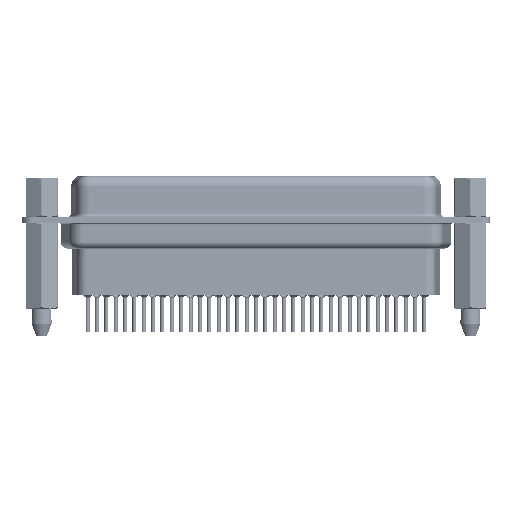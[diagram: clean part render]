
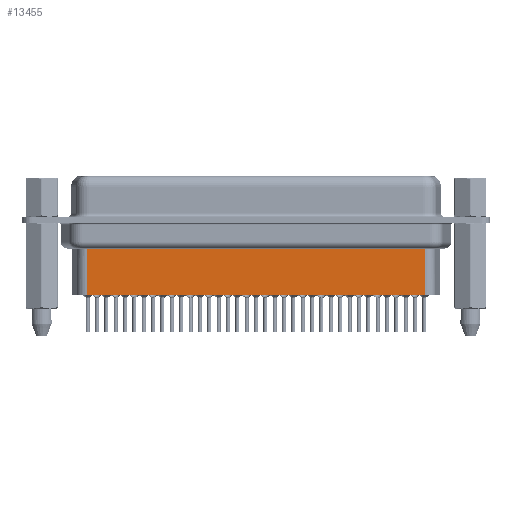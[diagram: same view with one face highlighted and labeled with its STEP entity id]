
A CAD part, front view. The second image highlights one B-rep face of the part: STEP entity #13455.
In plain terms, the highlighted planar face has unit normal (0, -1, 0).
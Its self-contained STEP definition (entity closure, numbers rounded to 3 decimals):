
#144 = CARTESIAN_POINT ( 'NONE',  ( 56.794, -3.5, -4.097 ) ) ;
#350 = VERTEX_POINT ( 'NONE', #13398 ) ;
#1258 = VECTOR ( 'NONE', #24046, 1000. ) ;
#1282 = DIRECTION ( 'NONE',  ( 1., 0., 0. ) ) ;
#3902 = DIRECTION ( 'NONE',  ( 0., 0., -1. ) ) ;
#7514 = EDGE_CURVE ( 'NONE', #37423, #31630, #21726, .T. ) ;
#7929 = AXIS2_PLACEMENT_3D ( 'NONE', #31589, #13810, #1282 ) ;
#12096 = LINE ( 'NONE', #15792, #1258 ) ;
#13398 = CARTESIAN_POINT ( 'NONE',  ( 6.706, -3.5, -11.15 ) ) ;
#13455 = ADVANCED_FACE ( 'NONE', ( #25570 ), #19672, .T. ) ;
#13810 = DIRECTION ( 'NONE',  ( 0., -1., 0. ) ) ;
#15675 = LINE ( 'NONE', #24492, #19943 ) ;
#15792 = CARTESIAN_POINT ( 'NONE',  ( 6.706, -3.5, -3.1 ) ) ;
#17318 = ORIENTED_EDGE ( 'NONE', *, *, #25133, .T. ) ;
#19672 = PLANE ( 'NONE',  #7929 ) ;
#19943 = VECTOR ( 'NONE', #21552, 1000. ) ;
#21325 = EDGE_LOOP ( 'NONE', ( #38346, #21705, #17318, #33571 ) ) ;
#21552 = DIRECTION ( 'NONE',  ( -1., 0., 0. ) ) ;
#21705 = ORIENTED_EDGE ( 'NONE', *, *, #23804, .T. ) ;
#21726 = LINE ( 'NONE', #36768, #24311 ) ;
#22037 = VERTEX_POINT ( 'NONE', #36247 ) ;
#22688 = VECTOR ( 'NONE', #36026, 1000. ) ;
#23804 = EDGE_CURVE ( 'NONE', #37423, #22037, #15675, .T. ) ;
#24046 = DIRECTION ( 'NONE',  ( 0., 0., -1. ) ) ;
#24311 = VECTOR ( 'NONE', #3902, 1000. ) ;
#24492 = CARTESIAN_POINT ( 'NONE',  ( 6.459, -3.5, -4.097 ) ) ;
#25133 = EDGE_CURVE ( 'NONE', #22037, #350, #12096, .T. ) ;
#25570 = FACE_OUTER_BOUND ( 'NONE', #21325, .T. ) ;
#27043 = CARTESIAN_POINT ( 'NONE',  ( 6.706, -3.5, -11.15 ) ) ;
#29711 = EDGE_CURVE ( 'NONE', #31630, #350, #36407, .T. ) ;
#30865 = CARTESIAN_POINT ( 'NONE',  ( 56.794, -3.5, -11.15 ) ) ;
#31589 = CARTESIAN_POINT ( 'NONE',  ( 6.706, -3.5, -3.1 ) ) ;
#31630 = VERTEX_POINT ( 'NONE', #30865 ) ;
#33571 = ORIENTED_EDGE ( 'NONE', *, *, #29711, .F. ) ;
#36026 = DIRECTION ( 'NONE',  ( -1., 0., 0. ) ) ;
#36247 = CARTESIAN_POINT ( 'NONE',  ( 6.706, -3.5, -4.097 ) ) ;
#36407 = LINE ( 'NONE', #27043, #22688 ) ;
#36768 = CARTESIAN_POINT ( 'NONE',  ( 56.794, -3.5, -3.1 ) ) ;
#37423 = VERTEX_POINT ( 'NONE', #144 ) ;
#38346 = ORIENTED_EDGE ( 'NONE', *, *, #7514, .F. ) ;
